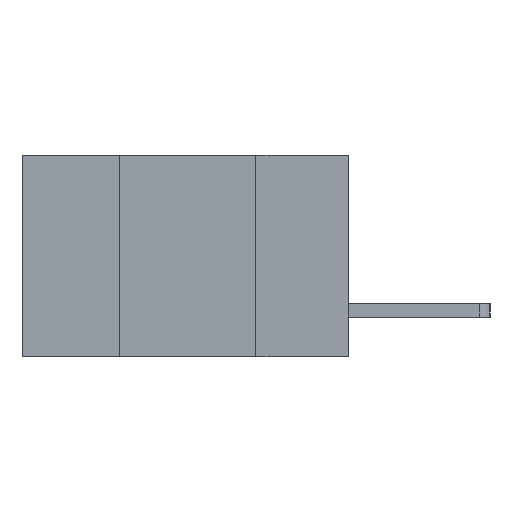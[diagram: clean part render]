
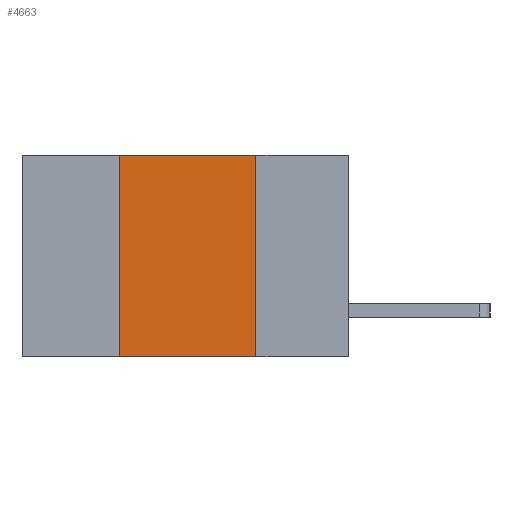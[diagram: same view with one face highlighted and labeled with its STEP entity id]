
A CAD part, left-side view. The second image highlights one B-rep face of the part: STEP entity #4663.
In plain terms, the highlighted planar face has unit normal (-1, 0, 0).
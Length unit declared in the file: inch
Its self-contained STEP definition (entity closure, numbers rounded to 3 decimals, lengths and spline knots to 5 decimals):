
#771 = ORIENTED_EDGE ( 'NONE', *, *, #5806, .F. ) ;
#1586 = VERTEX_POINT ( 'NONE', #6352 ) ;
#1750 = CARTESIAN_POINT ( 'NONE',  ( 0., 0.6, -0.37 ) ) ;
#2364 = VERTEX_POINT ( 'NONE', #7786 ) ;
#2426 = VECTOR ( 'NONE', #4446, 39.37008 ) ;
#2631 = VERTEX_POINT ( 'NONE', #5947 ) ;
#2780 = EDGE_CURVE ( 'NONE', #2364, #1586, #6424, .T. ) ;
#3145 = DIRECTION ( 'NONE',  ( 0., 0., 1. ) ) ;
#3172 = CARTESIAN_POINT ( 'NONE',  ( 0., 0.42, -0.37 ) ) ;
#3618 = FACE_OUTER_BOUND ( 'NONE', #8371, .T. ) ;
#4446 = DIRECTION ( 'NONE',  ( 0., -1., 0. ) ) ;
#4447 = DIRECTION ( 'NONE',  ( 0., 0., -1. ) ) ;
#4612 = VECTOR ( 'NONE', #6271, 39.37008 ) ;
#4634 = DIRECTION ( 'NONE',  ( 1., 0., 0. ) ) ;
#4661 = EDGE_CURVE ( 'NONE', #1586, #6673, #5831, .T. ) ;
#4663 = ADVANCED_FACE ( 'NONE', ( #3618 ), #4868, .F. ) ;
#4668 = CARTESIAN_POINT ( 'NONE',  ( 0., 0.6, 0. ) ) ;
#4868 = PLANE ( 'NONE',  #8192 ) ;
#5116 = CARTESIAN_POINT ( 'NONE',  ( 0., 0.17, -0.37 ) ) ;
#5289 = DIRECTION ( 'NONE',  ( 0., 0., -1. ) ) ;
#5556 = ORIENTED_EDGE ( 'NONE', *, *, #4661, .F. ) ;
#5703 = VECTOR ( 'NONE', #3145, 39.37008 ) ;
#5806 = EDGE_CURVE ( 'NONE', #2631, #2364, #7499, .T. ) ;
#5831 = LINE ( 'NONE', #5116, #7206 ) ;
#5947 = CARTESIAN_POINT ( 'NONE',  ( 0., 0.42, -0.37 ) ) ;
#6177 = LINE ( 'NONE', #1750, #2426 ) ;
#6271 = DIRECTION ( 'NONE',  ( 0., -1., 0. ) ) ;
#6352 = CARTESIAN_POINT ( 'NONE',  ( 0., 0.17, 0. ) ) ;
#6424 = LINE ( 'NONE', #7841, #4612 ) ;
#6673 = VERTEX_POINT ( 'NONE', #6941 ) ;
#6941 = CARTESIAN_POINT ( 'NONE',  ( 0., 0.17, -0.37 ) ) ;
#7058 = ORIENTED_EDGE ( 'NONE', *, *, #2780, .F. ) ;
#7206 = VECTOR ( 'NONE', #5289, 39.37008 ) ;
#7499 = LINE ( 'NONE', #3172, #5703 ) ;
#7786 = CARTESIAN_POINT ( 'NONE',  ( 0., 0.42, 0. ) ) ;
#7841 = CARTESIAN_POINT ( 'NONE',  ( 0., 0.6, 0. ) ) ;
#8192 = AXIS2_PLACEMENT_3D ( 'NONE', #4668, #4634, #4447 ) ;
#8308 = ORIENTED_EDGE ( 'NONE', *, *, #8597, .T. ) ;
#8371 = EDGE_LOOP ( 'NONE', ( #5556, #7058, #771, #8308 ) ) ;
#8597 = EDGE_CURVE ( 'NONE', #2631, #6673, #6177, .T. ) ;
